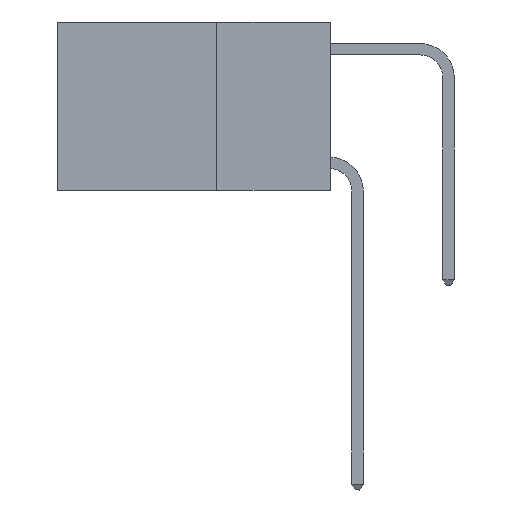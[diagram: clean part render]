
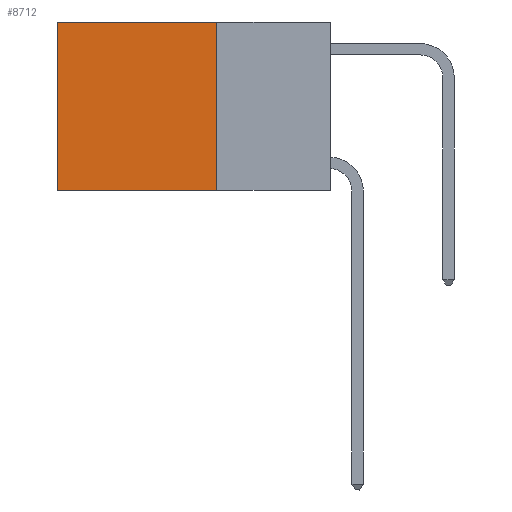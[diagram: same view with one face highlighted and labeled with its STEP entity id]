
A CAD part, left-side view. The second image highlights one B-rep face of the part: STEP entity #8712.
In plain terms, the highlighted planar face has unit normal (-1, 0, 0).
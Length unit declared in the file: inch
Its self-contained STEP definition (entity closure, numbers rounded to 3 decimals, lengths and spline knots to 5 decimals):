
#296 = CARTESIAN_POINT ( 'NONE',  ( 0.2625, 0.25, -0.37 ) ) ;
#1177 = DIRECTION ( 'NONE',  ( 1., 0., 0. ) ) ;
#3193 = VERTEX_POINT ( 'NONE', #18312 ) ;
#3687 = LINE ( 'NONE', #21574, #19374 ) ;
#4440 = VECTOR ( 'NONE', #10145, 39.37008 ) ;
#4597 = VECTOR ( 'NONE', #9055, 39.37008 ) ;
#5253 = LINE ( 'NONE', #23170, #4597 ) ;
#8454 = DIRECTION ( 'NONE',  ( 0., 1., 0. ) ) ;
#8712 = ADVANCED_FACE ( 'NONE', ( #13965 ), #21493, .F. ) ;
#8717 = EDGE_CURVE ( 'NONE', #3193, #12141, #3687, .T. ) ;
#9055 = DIRECTION ( 'NONE',  ( 0., 1., 0. ) ) ;
#9308 = EDGE_CURVE ( 'NONE', #9962, #3193, #5253, .T. ) ;
#9962 = VERTEX_POINT ( 'NONE', #15096 ) ;
#10145 = DIRECTION ( 'NONE',  ( 0., 0., -1. ) ) ;
#11029 = ORIENTED_EDGE ( 'NONE', *, *, #9308, .T. ) ;
#11943 = EDGE_LOOP ( 'NONE', ( #13165, #12854, #26078, #11029 ) ) ;
#12141 = VERTEX_POINT ( 'NONE', #20266 ) ;
#12353 = VECTOR ( 'NONE', #8454, 39.37008 ) ;
#12854 = ORIENTED_EDGE ( 'NONE', *, *, #25308, .F. ) ;
#12996 = VERTEX_POINT ( 'NONE', #18854 ) ;
#13000 = LINE ( 'NONE', #296, #12353 ) ;
#13165 = ORIENTED_EDGE ( 'NONE', *, *, #8717, .T. ) ;
#13484 = CARTESIAN_POINT ( 'NONE',  ( 0.2625, 0.25, 0. ) ) ;
#13965 = FACE_OUTER_BOUND ( 'NONE', #11943, .T. ) ;
#14232 = EDGE_CURVE ( 'NONE', #9962, #12996, #25269, .T. ) ;
#15096 = CARTESIAN_POINT ( 'NONE',  ( 0.2625, 0.25, 0. ) ) ;
#15510 = DIRECTION ( 'NONE',  ( 0., 0., -1. ) ) ;
#18312 = CARTESIAN_POINT ( 'NONE',  ( 0.2625, 0.6, 0. ) ) ;
#18360 = CARTESIAN_POINT ( 'NONE',  ( 0.2625, 0.25, 0. ) ) ;
#18854 = CARTESIAN_POINT ( 'NONE',  ( 0.2625, 0.25, -0.37 ) ) ;
#19374 = VECTOR ( 'NONE', #25381, 39.37008 ) ;
#20266 = CARTESIAN_POINT ( 'NONE',  ( 0.2625, 0.6, -0.37 ) ) ;
#21493 = PLANE ( 'NONE',  #26080 ) ;
#21574 = CARTESIAN_POINT ( 'NONE',  ( 0.2625, 0.6, 0. ) ) ;
#23170 = CARTESIAN_POINT ( 'NONE',  ( 0.2625, 0.25, 0. ) ) ;
#25269 = LINE ( 'NONE', #18360, #4440 ) ;
#25308 = EDGE_CURVE ( 'NONE', #12996, #12141, #13000, .T. ) ;
#25381 = DIRECTION ( 'NONE',  ( 0., 0., -1. ) ) ;
#26078 = ORIENTED_EDGE ( 'NONE', *, *, #14232, .F. ) ;
#26080 = AXIS2_PLACEMENT_3D ( 'NONE', #13484, #1177, #15510 ) ;
